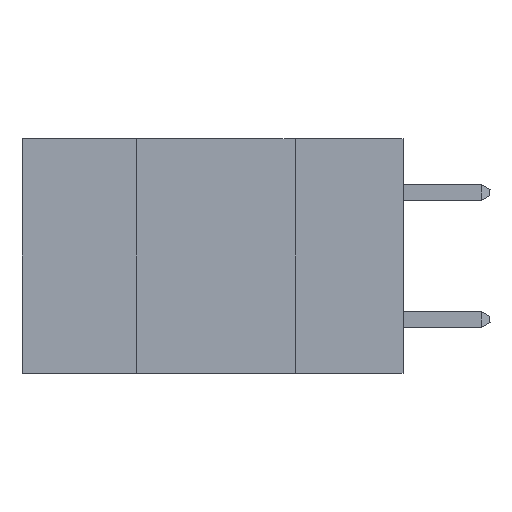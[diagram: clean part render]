
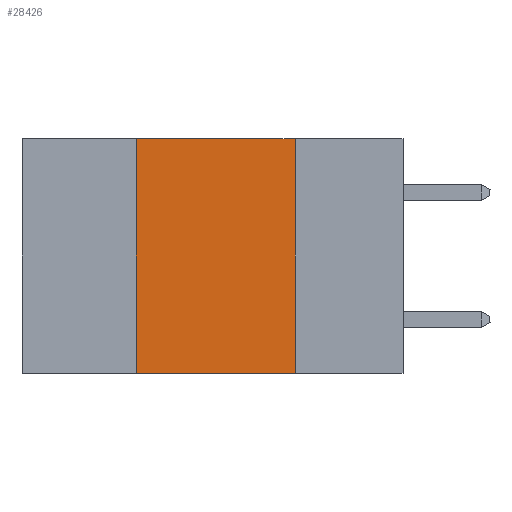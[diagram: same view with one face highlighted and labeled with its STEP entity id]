
A CAD part, left-side view. The second image highlights one B-rep face of the part: STEP entity #28426.
In plain terms, the highlighted planar face has unit normal (-1, 0, 0).
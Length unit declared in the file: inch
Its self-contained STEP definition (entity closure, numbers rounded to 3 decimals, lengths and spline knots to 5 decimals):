
#1342 = DIRECTION ( 'NONE',  ( 0., -1., 0. ) ) ;
#1970 = FACE_OUTER_BOUND ( 'NONE', #19938, .T. ) ;
#2827 = VERTEX_POINT ( 'NONE', #24612 ) ;
#3954 = DIRECTION ( 'NONE',  ( 0., 0., 1. ) ) ;
#4323 = CARTESIAN_POINT ( 'NONE',  ( 0., 0.17, 0. ) ) ;
#4541 = DIRECTION ( 'NONE',  ( 0., -1., 0. ) ) ;
#5575 = VERTEX_POINT ( 'NONE', #23459 ) ;
#6792 = PLANE ( 'NONE',  #23164 ) ;
#7477 = EDGE_CURVE ( 'NONE', #5575, #2827, #28708, .T. ) ;
#7769 = EDGE_CURVE ( 'NONE', #26751, #10673, #16531, .T. ) ;
#7866 = LINE ( 'NONE', #21932, #15951 ) ;
#10673 = VERTEX_POINT ( 'NONE', #4323 ) ;
#13249 = ORIENTED_EDGE ( 'NONE', *, *, #7769, .F. ) ;
#15426 = EDGE_CURVE ( 'NONE', #5575, #26751, #18251, .T. ) ;
#15951 = VECTOR ( 'NONE', #26285, 39.37008 ) ;
#16349 = DIRECTION ( 'NONE',  ( 1., 0., 0. ) ) ;
#16531 = LINE ( 'NONE', #29361, #18778 ) ;
#17076 = EDGE_CURVE ( 'NONE', #10673, #2827, #7866, .T. ) ;
#18251 = LINE ( 'NONE', #27115, #28901 ) ;
#18333 = CARTESIAN_POINT ( 'NONE',  ( 0., 0.6, -0.37 ) ) ;
#18776 = CARTESIAN_POINT ( 'NONE',  ( 0., 0.42, 0. ) ) ;
#18778 = VECTOR ( 'NONE', #1342, 39.37008 ) ;
#19938 = EDGE_LOOP ( 'NONE', ( #20907, #13249, #24795, #27556 ) ) ;
#20907 = ORIENTED_EDGE ( 'NONE', *, *, #17076, .F. ) ;
#21363 = VECTOR ( 'NONE', #4541, 39.37008 ) ;
#21932 = CARTESIAN_POINT ( 'NONE',  ( 0., 0.17, 0. ) ) ;
#23164 = AXIS2_PLACEMENT_3D ( 'NONE', #25956, #16349, #25862 ) ;
#23459 = CARTESIAN_POINT ( 'NONE',  ( 0., 0.42, -0.37 ) ) ;
#24612 = CARTESIAN_POINT ( 'NONE',  ( 0., 0.17, -0.37 ) ) ;
#24795 = ORIENTED_EDGE ( 'NONE', *, *, #15426, .F. ) ;
#25862 = DIRECTION ( 'NONE',  ( 0., 0., -1. ) ) ;
#25956 = CARTESIAN_POINT ( 'NONE',  ( 0., 0.6, 0. ) ) ;
#26285 = DIRECTION ( 'NONE',  ( 0., 0., -1. ) ) ;
#26751 = VERTEX_POINT ( 'NONE', #18776 ) ;
#27115 = CARTESIAN_POINT ( 'NONE',  ( 0., 0.42, 0. ) ) ;
#27556 = ORIENTED_EDGE ( 'NONE', *, *, #7477, .T. ) ;
#28426 = ADVANCED_FACE ( 'NONE', ( #1970 ), #6792, .F. ) ;
#28708 = LINE ( 'NONE', #18333, #21363 ) ;
#28901 = VECTOR ( 'NONE', #3954, 39.37008 ) ;
#29361 = CARTESIAN_POINT ( 'NONE',  ( 0., 0.6, 0. ) ) ;
